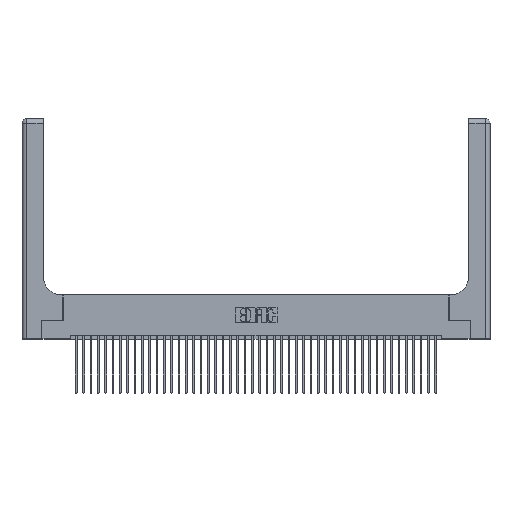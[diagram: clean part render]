
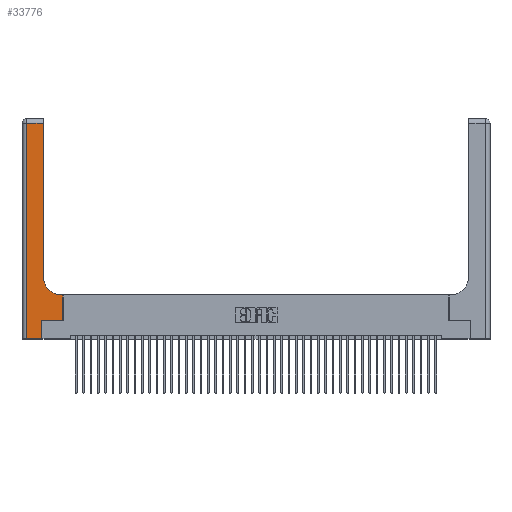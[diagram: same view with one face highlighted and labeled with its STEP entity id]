
A CAD part, top view. The second image highlights one B-rep face of the part: STEP entity #33776.
In plain terms, the highlighted planar face has unit normal (0, 0, 1).
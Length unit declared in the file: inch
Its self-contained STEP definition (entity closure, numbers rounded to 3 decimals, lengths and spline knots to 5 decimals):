
#320 = CARTESIAN_POINT ( 'NONE',  ( 0.2915, 3., 0.37 ) ) ;
#1754 = VERTEX_POINT ( 'NONE', #34311 ) ;
#1809 = EDGE_CURVE ( 'NONE', #29676, #1754, #31560, .T. ) ;
#2460 = VERTEX_POINT ( 'NONE', #27585 ) ;
#3914 = VECTOR ( 'NONE', #13836, 39.37008 ) ;
#4527 = ORIENTED_EDGE ( 'NONE', *, *, #1809, .T. ) ;
#4604 = VERTEX_POINT ( 'NONE', #22295 ) ;
#4675 = VECTOR ( 'NONE', #21525, 39.37008 ) ;
#4902 = DIRECTION ( 'NONE',  ( 0., 0., -1. ) ) ;
#4903 = VECTOR ( 'NONE', #13839, 39.37008 ) ;
#4946 = VERTEX_POINT ( 'NONE', #27536 ) ;
#5078 = CARTESIAN_POINT ( 'NONE',  ( 0.5585, 0.25, 0.37 ) ) ;
#5376 = CARTESIAN_POINT ( 'NONE',  ( 0.06, 3., 0.37 ) ) ;
#5528 = ORIENTED_EDGE ( 'NONE', *, *, #38941, .T. ) ;
#5883 = VERTEX_POINT ( 'NONE', #32171 ) ;
#5919 = EDGE_CURVE ( 'NONE', #9500, #37137, #33876, .T. ) ;
#6128 = VECTOR ( 'NONE', #12937, 39.37008 ) ;
#6712 = CARTESIAN_POINT ( 'NONE',  ( 0., 3., 0.37 ) ) ;
#7104 = ORIENTED_EDGE ( 'NONE', *, *, #40854, .T. ) ;
#7665 = EDGE_CURVE ( 'NONE', #37137, #5883, #24369, .T. ) ;
#8774 = CARTESIAN_POINT ( 'NONE',  ( 0.269, 0.25, 0.37 ) ) ;
#8907 = DIRECTION ( 'NONE',  ( -1., 0., 0. ) ) ;
#9500 = VERTEX_POINT ( 'NONE', #10019 ) ;
#9806 = VECTOR ( 'NONE', #8907, 39.37008 ) ;
#10019 = CARTESIAN_POINT ( 'NONE',  ( 0.06, 2.94, 0.37 ) ) ;
#10446 = CARTESIAN_POINT ( 'NONE',  ( 0.5585, 0.25, 0.37 ) ) ;
#12936 = LINE ( 'NONE', #320, #3914 ) ;
#12937 = DIRECTION ( 'NONE',  ( 0., 1., 0. ) ) ;
#13836 = DIRECTION ( 'NONE',  ( 0., 1., 0. ) ) ;
#13839 = DIRECTION ( 'NONE',  ( 0., 1., 0. ) ) ;
#14232 = ORIENTED_EDGE ( 'NONE', *, *, #34189, .T. ) ;
#15525 = CARTESIAN_POINT ( 'NONE',  ( 0.06, 0., 0.37 ) ) ;
#15552 = AXIS2_PLACEMENT_3D ( 'NONE', #6712, #16946, #40180 ) ;
#16946 = DIRECTION ( 'NONE',  ( 0., 0., -1. ) ) ;
#17275 = ORIENTED_EDGE ( 'NONE', *, *, #39938, .T. ) ;
#18123 = CARTESIAN_POINT ( 'NONE',  ( 0.2915, 0.6, 0.37 ) ) ;
#18773 = AXIS2_PLACEMENT_3D ( 'NONE', #25157, #4902, #28535 ) ;
#19185 = ORIENTED_EDGE ( 'NONE', *, *, #5919, .T. ) ;
#20196 = EDGE_CURVE ( 'NONE', #1754, #4946, #41385, .T. ) ;
#20768 = ORIENTED_EDGE ( 'NONE', *, *, #20196, .T. ) ;
#21234 = VECTOR ( 'NONE', #42071, 39.37008 ) ;
#21525 = DIRECTION ( 'NONE',  ( -1., 0., 0. ) ) ;
#22254 = CARTESIAN_POINT ( 'NONE',  ( 0., 0., 0.37 ) ) ;
#22295 = CARTESIAN_POINT ( 'NONE',  ( 0.2915, 2.94, 0.37 ) ) ;
#22625 = FACE_OUTER_BOUND ( 'NONE', #39423, .T. ) ;
#23123 = CARTESIAN_POINT ( 'NONE',  ( 0.269, 0., 0.37 ) ) ;
#23325 = CARTESIAN_POINT ( 'NONE',  ( 0.5585, 0.6, 0.37 ) ) ;
#23636 = VECTOR ( 'NONE', #32300, 39.37008 ) ;
#24369 = LINE ( 'NONE', #22254, #21234 ) ;
#25157 = CARTESIAN_POINT ( 'NONE',  ( 0.5415, 0.85, 0.37 ) ) ;
#25735 = CARTESIAN_POINT ( 'NONE',  ( 0., 2.94, 0.37 ) ) ;
#25842 = EDGE_CURVE ( 'NONE', #5883, #2460, #40617, .T. ) ;
#26843 = ORIENTED_EDGE ( 'NONE', *, *, #7665, .T. ) ;
#27536 = CARTESIAN_POINT ( 'NONE',  ( 0.2915, 0.85, 0.37 ) ) ;
#27585 = CARTESIAN_POINT ( 'NONE',  ( 0.269, 0.25, 0.37 ) ) ;
#28535 = DIRECTION ( 'NONE',  ( 1., 0., 0. ) ) ;
#29676 = VERTEX_POINT ( 'NONE', #23325 ) ;
#29738 = LINE ( 'NONE', #10446, #4903 ) ;
#30532 = VERTEX_POINT ( 'NONE', #5078 ) ;
#31560 = LINE ( 'NONE', #18123, #4675 ) ;
#31841 = VECTOR ( 'NONE', #35612, 39.37008 ) ;
#32171 = CARTESIAN_POINT ( 'NONE',  ( 0.269, 0., 0.37 ) ) ;
#32300 = DIRECTION ( 'NONE',  ( 1., 0., 0. ) ) ;
#33776 = ADVANCED_FACE ( 'NONE', ( #22625 ), #36898, .F. ) ;
#33876 = LINE ( 'NONE', #5376, #31841 ) ;
#34189 = EDGE_CURVE ( 'NONE', #2460, #30532, #41194, .T. ) ;
#34311 = CARTESIAN_POINT ( 'NONE',  ( 0.5415, 0.6, 0.37 ) ) ;
#34431 = LINE ( 'NONE', #25735, #9806 ) ;
#35612 = DIRECTION ( 'NONE',  ( 0., -1., 0. ) ) ;
#36898 = PLANE ( 'NONE',  #15552 ) ;
#37137 = VERTEX_POINT ( 'NONE', #15525 ) ;
#38941 = EDGE_CURVE ( 'NONE', #4604, #9500, #34431, .T. ) ;
#39423 = EDGE_LOOP ( 'NONE', ( #17275, #5528, #19185, #26843, #42387, #14232, #7104, #4527, #20768 ) ) ;
#39938 = EDGE_CURVE ( 'NONE', #4946, #4604, #12936, .T. ) ;
#40180 = DIRECTION ( 'NONE',  ( -1., 0., 0. ) ) ;
#40617 = LINE ( 'NONE', #23123, #6128 ) ;
#40854 = EDGE_CURVE ( 'NONE', #30532, #29676, #29738, .T. ) ;
#41194 = LINE ( 'NONE', #8774, #23636 ) ;
#41385 = CIRCLE ( 'NONE', #18773, 0.25 ) ;
#42071 = DIRECTION ( 'NONE',  ( 1., 0., 0. ) ) ;
#42387 = ORIENTED_EDGE ( 'NONE', *, *, #25842, .T. ) ;
